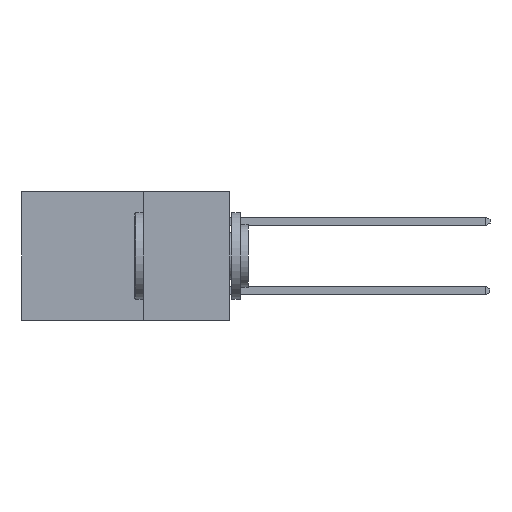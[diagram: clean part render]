
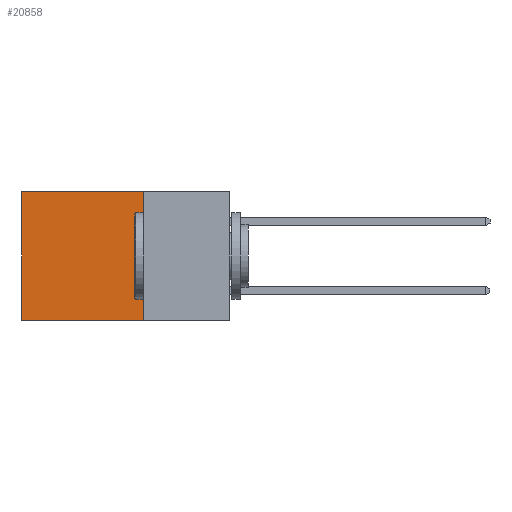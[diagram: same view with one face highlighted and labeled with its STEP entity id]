
A CAD part, left-side view. The second image highlights one B-rep face of the part: STEP entity #20858.
In plain terms, the highlighted planar face has unit normal (-1, 0, 0).
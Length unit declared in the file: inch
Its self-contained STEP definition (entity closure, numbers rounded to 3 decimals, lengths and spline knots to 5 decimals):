
#2290 = CARTESIAN_POINT ( 'NONE',  ( 0.298, 0.25, 0. ) ) ;
#3565 = VECTOR ( 'NONE', #4631, 39.37008 ) ;
#4380 = DIRECTION ( 'NONE',  ( 0., 0., -1. ) ) ;
#4631 = DIRECTION ( 'NONE',  ( 0., 1., 0. ) ) ;
#5723 = VERTEX_POINT ( 'NONE', #7222 ) ;
#6418 = EDGE_CURVE ( 'NONE', #10987, #5723, #28706, .T. ) ;
#6627 = PLANE ( 'NONE',  #10211 ) ;
#7222 = CARTESIAN_POINT ( 'NONE',  ( 0.298, 0.25, -0.37 ) ) ;
#8285 = LINE ( 'NONE', #29271, #19663 ) ;
#9106 = CARTESIAN_POINT ( 'NONE',  ( 0.298, 0.25, -0.37 ) ) ;
#9761 = LINE ( 'NONE', #2290, #3565 ) ;
#10211 = AXIS2_PLACEMENT_3D ( 'NONE', #13586, #29199, #15894 ) ;
#10416 = ORIENTED_EDGE ( 'NONE', *, *, #6418, .F. ) ;
#10987 = VERTEX_POINT ( 'NONE', #17242 ) ;
#11703 = VECTOR ( 'NONE', #18255, 39.37008 ) ;
#12401 = LINE ( 'NONE', #9106, #11703 ) ;
#13586 = CARTESIAN_POINT ( 'NONE',  ( 0.298, 0.25, 0. ) ) ;
#13688 = ORIENTED_EDGE ( 'NONE', *, *, #20898, .F. ) ;
#13887 = EDGE_LOOP ( 'NONE', ( #27064, #13688, #10416, #14664 ) ) ;
#14079 = VERTEX_POINT ( 'NONE', #19466 ) ;
#14664 = ORIENTED_EDGE ( 'NONE', *, *, #23364, .T. ) ;
#15894 = DIRECTION ( 'NONE',  ( 0., 0., -1. ) ) ;
#16057 = DIRECTION ( 'NONE',  ( 0., 0., -1. ) ) ;
#16902 = VECTOR ( 'NONE', #4380, 39.37008 ) ;
#17242 = CARTESIAN_POINT ( 'NONE',  ( 0.298, 0.25, 0. ) ) ;
#18255 = DIRECTION ( 'NONE',  ( 0., 1., 0. ) ) ;
#18509 = CARTESIAN_POINT ( 'NONE',  ( 0.298, 0.25, 0. ) ) ;
#19143 = FACE_OUTER_BOUND ( 'NONE', #13887, .T. ) ;
#19466 = CARTESIAN_POINT ( 'NONE',  ( 0.298, 0.6, 0. ) ) ;
#19663 = VECTOR ( 'NONE', #16057, 39.37008 ) ;
#20858 = ADVANCED_FACE ( 'NONE', ( #19143 ), #6627, .F. ) ;
#20898 = EDGE_CURVE ( 'NONE', #5723, #21233, #12401, .T. ) ;
#21233 = VERTEX_POINT ( 'NONE', #21627 ) ;
#21627 = CARTESIAN_POINT ( 'NONE',  ( 0.298, 0.6, -0.37 ) ) ;
#23364 = EDGE_CURVE ( 'NONE', #10987, #14079, #9761, .T. ) ;
#23870 = EDGE_CURVE ( 'NONE', #14079, #21233, #8285, .T. ) ;
#27064 = ORIENTED_EDGE ( 'NONE', *, *, #23870, .T. ) ;
#28706 = LINE ( 'NONE', #18509, #16902 ) ;
#29199 = DIRECTION ( 'NONE',  ( 1., 0., 0. ) ) ;
#29271 = CARTESIAN_POINT ( 'NONE',  ( 0.298, 0.6, 0. ) ) ;
